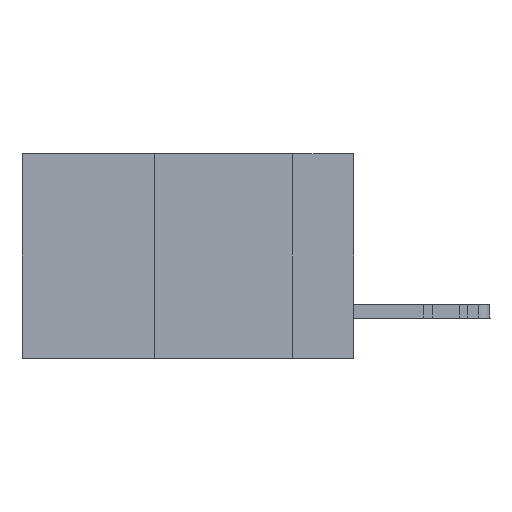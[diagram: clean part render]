
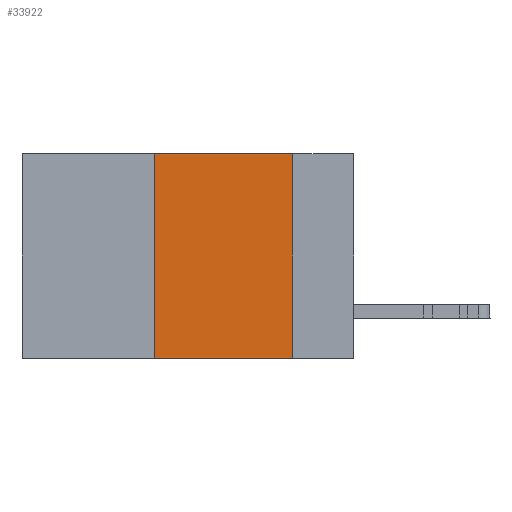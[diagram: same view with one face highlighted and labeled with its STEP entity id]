
A CAD part, left-side view. The second image highlights one B-rep face of the part: STEP entity #33922.
In plain terms, the highlighted planar face has unit normal (-1, 0, 0).
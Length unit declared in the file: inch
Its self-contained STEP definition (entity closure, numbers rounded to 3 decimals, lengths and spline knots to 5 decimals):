
#1790 = VERTEX_POINT ( 'NONE', #25028 ) ;
#3784 = EDGE_CURVE ( 'NONE', #24091, #20260, #34003, .T. ) ;
#4430 = EDGE_CURVE ( 'NONE', #1790, #8385, #6066, .T. ) ;
#5844 = DIRECTION ( 'NONE',  ( 0., -1., 0. ) ) ;
#5896 = DIRECTION ( 'NONE',  ( 0., 0., 1. ) ) ;
#6066 = LINE ( 'NONE', #40407, #39448 ) ;
#6212 = CARTESIAN_POINT ( 'NONE',  ( 0., 0.11, 0. ) ) ;
#6355 = LINE ( 'NONE', #33670, #22021 ) ;
#7533 = DIRECTION ( 'NONE',  ( 0., 0., -1. ) ) ;
#7582 = CARTESIAN_POINT ( 'NONE',  ( 0., 0.6, 0. ) ) ;
#8385 = VERTEX_POINT ( 'NONE', #6212 ) ;
#10885 = EDGE_CURVE ( 'NONE', #8385, #20260, #42313, .T. ) ;
#11493 = ORIENTED_EDGE ( 'NONE', *, *, #4430, .F. ) ;
#16353 = CARTESIAN_POINT ( 'NONE',  ( 0., 0.36, -0.37 ) ) ;
#16656 = ORIENTED_EDGE ( 'NONE', *, *, #10885, .F. ) ;
#16825 = DIRECTION ( 'NONE',  ( 0., -1., 0. ) ) ;
#17283 = EDGE_CURVE ( 'NONE', #24091, #1790, #6355, .T. ) ;
#17447 = ORIENTED_EDGE ( 'NONE', *, *, #3784, .T. ) ;
#17894 = ORIENTED_EDGE ( 'NONE', *, *, #17283, .F. ) ;
#20260 = VERTEX_POINT ( 'NONE', #39823 ) ;
#21115 = PLANE ( 'NONE',  #32461 ) ;
#21336 = DIRECTION ( 'NONE',  ( 1., 0., 0. ) ) ;
#22021 = VECTOR ( 'NONE', #5896, 39.37008 ) ;
#22171 = VECTOR ( 'NONE', #7533, 39.37008 ) ;
#24091 = VERTEX_POINT ( 'NONE', #16353 ) ;
#24100 = VECTOR ( 'NONE', #16825, 39.37008 ) ;
#24724 = FACE_OUTER_BOUND ( 'NONE', #32783, .T. ) ;
#25028 = CARTESIAN_POINT ( 'NONE',  ( 0., 0.36, 0. ) ) ;
#28959 = CARTESIAN_POINT ( 'NONE',  ( 0., 0.11, 0. ) ) ;
#31066 = CARTESIAN_POINT ( 'NONE',  ( 0., 0.6, -0.37 ) ) ;
#32461 = AXIS2_PLACEMENT_3D ( 'NONE', #7582, #21336, #35119 ) ;
#32783 = EDGE_LOOP ( 'NONE', ( #16656, #11493, #17894, #17447 ) ) ;
#33670 = CARTESIAN_POINT ( 'NONE',  ( 0., 0.36, 0. ) ) ;
#33922 = ADVANCED_FACE ( 'NONE', ( #24724 ), #21115, .F. ) ;
#34003 = LINE ( 'NONE', #31066, #24100 ) ;
#35119 = DIRECTION ( 'NONE',  ( 0., 0., -1. ) ) ;
#39448 = VECTOR ( 'NONE', #5844, 39.37008 ) ;
#39823 = CARTESIAN_POINT ( 'NONE',  ( 0., 0.11, -0.37 ) ) ;
#40407 = CARTESIAN_POINT ( 'NONE',  ( 0., 0.6, 0. ) ) ;
#42313 = LINE ( 'NONE', #28959, #22171 ) ;
